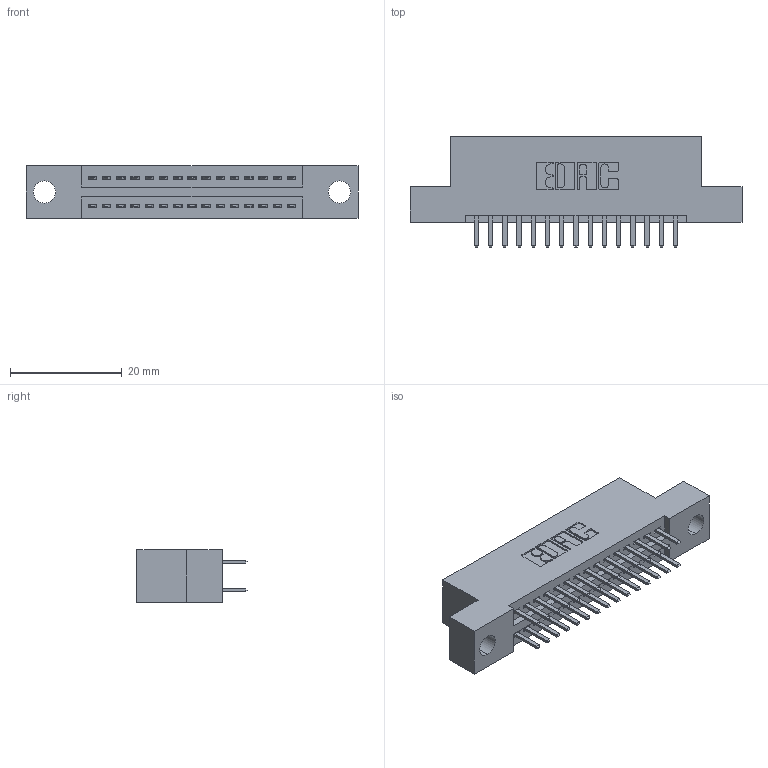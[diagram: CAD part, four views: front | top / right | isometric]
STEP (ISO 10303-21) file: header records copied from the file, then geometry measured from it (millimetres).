
FILE_DESCRIPTION (( 'STEP AP203' ), '1' );
FILE_NAME ('345-030-520-204.STEP', '2018-08-23T03:26:17', ( '' ), ( '' ), 'SwSTEP 2.0', 'SolidWorks 2016', '' );
FILE_SCHEMA (( 'CONFIG_CONTROL_DESIGN' ));
Length unit declared in the file: inch
Products named in the file (3): 345 Part_Flush Mounting Lugs - 0.156 Dia-TH; 345-292-001_345-293-120; 345-030-520-204
Assembly tree (31 placements, depth 2):
  345-030-520-204
    345 Part_Flush Mounting Lugs - 0.156 Dia-TH
    345-292-001_345-293-120  x30
Bounding box: 59.31 x 19.68 x 9.4 mm (x, y, z)
Volume: 5409.7 mm3; surface area: 7260.6 mm2
Topology: 31 solids, 31 shells, 1746 faces, 5051 edges, 3286 vertices
Faces by surface type: plane 1130, cylinder 616
Entity records: 15521 total; most frequent: CARTESIAN_POINT 2640, ORIENTED_EDGE 2562, DIRECTION 2349, EDGE_CURVE 1281, LINE 1085, VECTOR 1085, VERTEX_POINT 850, AXIS2_PLACEMENT_3D 632
